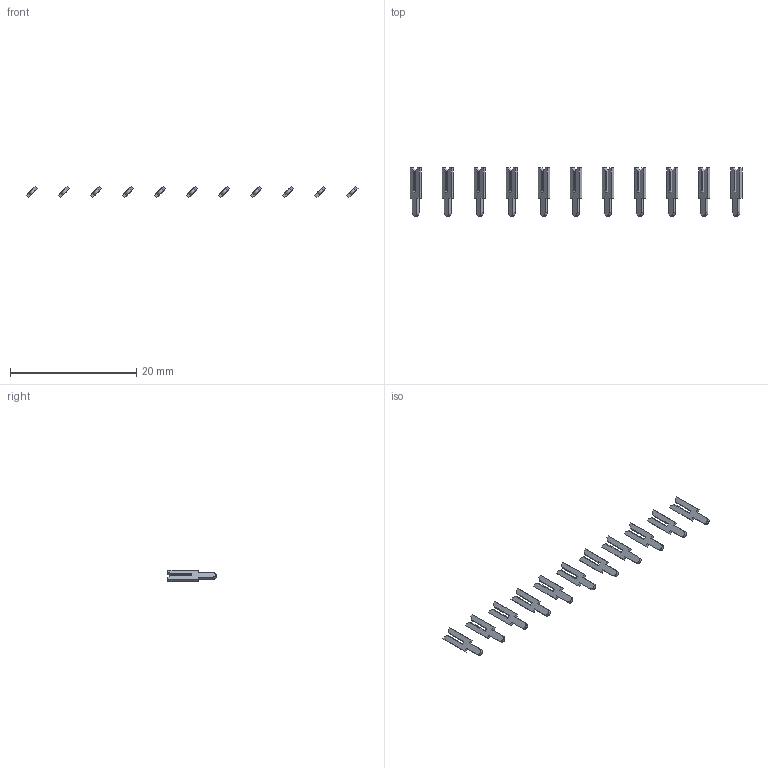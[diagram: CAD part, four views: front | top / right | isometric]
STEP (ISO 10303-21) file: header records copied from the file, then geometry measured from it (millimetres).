
FILE_DESCRIPTION (( 'STEP AP203' ), '1' );
FILE_NAME ('106-011-253-200.STEP', '2020-04-16T18:29:50', ( '' ), ( '' ), 'SwSTEP 2.0', 'SolidWorks 2016', '' );
FILE_SCHEMA (( 'CONFIG_CONTROL_DESIGN' ));
Length unit declared in the file: inch
Products named in the file (2): 106-011-253-200; 100-290-001_100-290-253
Assembly tree (11 placements, depth 2):
  106-011-253-200
    100-290-001_100-290-253  x11
Bounding box: 52.6 x 7.62 x 1.8 mm (x, y, z)
Volume: 60.7 mm3; surface area: 378.5 mm2
Topology: 11 solids, 11 shells, 220 faces, 594 edges, 396 vertices
Faces by surface type: plane 209, cylinder 11
Entity records: 1140 total; most frequent: DIRECTION 124, CARTESIAN_POINT 124, ORIENTED_EDGE 108, EDGE_CURVE 54, LINE 52, VECTOR 52, VERTEX_POINT 36, AXIS2_PLACEMENT_3D 36
